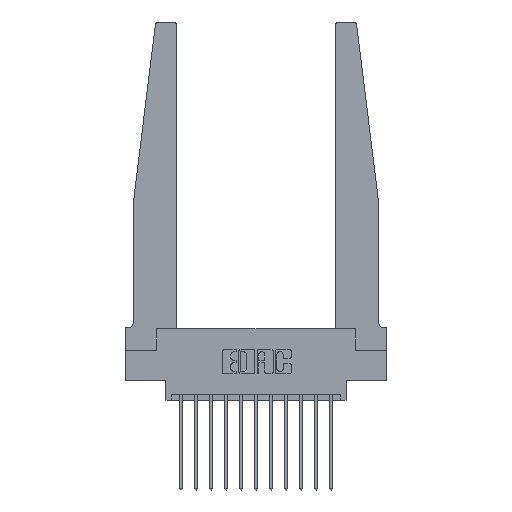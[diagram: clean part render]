
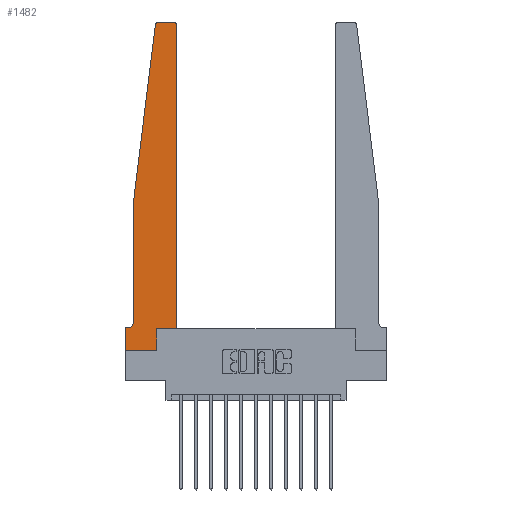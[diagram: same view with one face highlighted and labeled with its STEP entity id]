
A CAD part, top view. The second image highlights one B-rep face of the part: STEP entity #1482.
In plain terms, the highlighted planar face has unit normal (0, 0, 1).
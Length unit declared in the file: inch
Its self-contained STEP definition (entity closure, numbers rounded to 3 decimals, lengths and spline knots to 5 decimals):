
#38 = DIRECTION ( 'NONE',  ( 0., 0., 1. ) ) ;
#149 = ORIENTED_EDGE ( 'NONE', *, *, #4136, .T. ) ;
#203 = ORIENTED_EDGE ( 'NONE', *, *, #2887, .T. ) ;
#298 = ORIENTED_EDGE ( 'NONE', *, *, #16322, .T. ) ;
#369 = VECTOR ( 'NONE', #16697, 39.37008 ) ;
#582 = EDGE_CURVE ( 'NONE', #7267, #15739, #4285, .T. ) ;
#693 = EDGE_LOOP ( 'NONE', ( #4557, #298, #203, #1766, #14340, #6751, #10985, #16572, #149, #13660, #3062, #7093 ) ) ;
#736 = CIRCLE ( 'NONE', #2923, 0.05 ) ;
#879 = VERTEX_POINT ( 'NONE', #2829 ) ;
#1478 = CARTESIAN_POINT ( 'NONE',  ( 0.27653, 2.72, 0.37 ) ) ;
#1482 = ADVANCED_FACE ( 'NONE', ( #11853 ), #2599, .T. ) ;
#1578 = CARTESIAN_POINT ( 'NONE',  ( 0.24675, 2.72367, 0.37 ) ) ;
#1766 = ORIENTED_EDGE ( 'NONE', *, *, #582, .T. ) ;
#1962 = EDGE_CURVE ( 'NONE', #14315, #5229, #7698, .T. ) ;
#2391 = CARTESIAN_POINT ( 'NONE',  ( 0.015, 0.2375, 0.37 ) ) ;
#2501 = DIRECTION ( 'NONE',  ( 0., -1., 0. ) ) ;
#2599 = PLANE ( 'NONE',  #12465 ) ;
#2829 = CARTESIAN_POINT ( 'NONE',  ( 0.425, 0.18, 0.37 ) ) ;
#2849 = CARTESIAN_POINT ( 'NONE',  ( 0., 0.1875, 0.37 ) ) ;
#2887 = EDGE_CURVE ( 'NONE', #5390, #7267, #6261, .T. ) ;
#2923 = AXIS2_PLACEMENT_3D ( 'NONE', #2391, #7823, #10349 ) ;
#3027 = EDGE_CURVE ( 'NONE', #13052, #7630, #5092, .T. ) ;
#3062 = ORIENTED_EDGE ( 'NONE', *, *, #7537, .T. ) ;
#3632 = VERTEX_POINT ( 'NONE', #8326 ) ;
#3719 = LINE ( 'NONE', #8843, #8443 ) ;
#3731 = CARTESIAN_POINT ( 'NONE',  ( 0., 0., 0.37 ) ) ;
#4136 = EDGE_CURVE ( 'NONE', #5229, #7409, #14974, .T. ) ;
#4186 = DIRECTION ( 'NONE',  ( 0., 0., 1. ) ) ;
#4270 = CARTESIAN_POINT ( 'NONE',  ( 0.065, 0.1875, 0.37 ) ) ;
#4285 = LINE ( 'NONE', #14522, #10588 ) ;
#4311 = VECTOR ( 'NONE', #8189, 39.37008 ) ;
#4557 = ORIENTED_EDGE ( 'NONE', *, *, #11952, .T. ) ;
#4696 = CARTESIAN_POINT ( 'NONE',  ( 0.395, 2.75, 0.37 ) ) ;
#4885 = EDGE_CURVE ( 'NONE', #13196, #3632, #11730, .T. ) ;
#5019 = LINE ( 'NONE', #3731, #9753 ) ;
#5092 = CIRCLE ( 'NONE', #9356, 0.03 ) ;
#5199 = DIRECTION ( 'NONE',  ( 0., 0., 1. ) ) ;
#5229 = VERTEX_POINT ( 'NONE', #8824 ) ;
#5390 = VERTEX_POINT ( 'NONE', #1578 ) ;
#5505 = CARTESIAN_POINT ( 'NONE',  ( 0.425, 2.72, 0.37 ) ) ;
#6079 = CARTESIAN_POINT ( 'NONE',  ( 0., 0., 0.37 ) ) ;
#6261 = LINE ( 'NONE', #11383, #14456 ) ;
#6651 = DIRECTION ( 'NONE',  ( 0., 1., 0. ) ) ;
#6682 = DIRECTION ( 'NONE',  ( 1., 0., 0. ) ) ;
#6751 = ORIENTED_EDGE ( 'NONE', *, *, #4885, .T. ) ;
#6905 = CARTESIAN_POINT ( 'NONE',  ( 0.425, 0.18, 0.37 ) ) ;
#7093 = ORIENTED_EDGE ( 'NONE', *, *, #3027, .T. ) ;
#7267 = VERTEX_POINT ( 'NONE', #12842 ) ;
#7409 = VERTEX_POINT ( 'NONE', #8949 ) ;
#7537 = EDGE_CURVE ( 'NONE', #879, #13052, #15568, .T. ) ;
#7579 = CARTESIAN_POINT ( 'NONE',  ( 0.2605, 0.18, 0.37 ) ) ;
#7630 = VERTEX_POINT ( 'NONE', #4696 ) ;
#7698 = LINE ( 'NONE', #11559, #369 ) ;
#7778 = VECTOR ( 'NONE', #15057, 39.37008 ) ;
#7823 = DIRECTION ( 'NONE',  ( 0., 0., -1. ) ) ;
#8189 = DIRECTION ( 'NONE',  ( -1., 0., 0. ) ) ;
#8197 = VERTEX_POINT ( 'NONE', #10667 ) ;
#8326 = CARTESIAN_POINT ( 'NONE',  ( 0., 0.1875, 0.37 ) ) ;
#8443 = VECTOR ( 'NONE', #16583, 39.37008 ) ;
#8824 = CARTESIAN_POINT ( 'NONE',  ( 0.2605, 0., 0.37 ) ) ;
#8843 = CARTESIAN_POINT ( 'NONE',  ( 0.25, 2.75, 0.37 ) ) ;
#8949 = CARTESIAN_POINT ( 'NONE',  ( 0.2605, 0.18, 0.37 ) ) ;
#9166 = CARTESIAN_POINT ( 'NONE',  ( 0.425, 0.18, 0.37 ) ) ;
#9193 = CARTESIAN_POINT ( 'NONE',  ( 0.065, 0.2375, 0.37 ) ) ;
#9356 = AXIS2_PLACEMENT_3D ( 'NONE', #11712, #38, #6682 ) ;
#9753 = VECTOR ( 'NONE', #2501, 39.37008 ) ;
#10349 = DIRECTION ( 'NONE',  ( -1., 0., 0. ) ) ;
#10469 = CARTESIAN_POINT ( 'NONE',  ( 0.015, 0.1875, 0.37 ) ) ;
#10473 = EDGE_CURVE ( 'NONE', #7409, #879, #16117, .T. ) ;
#10588 = VECTOR ( 'NONE', #14607, 39.37008 ) ;
#10667 = CARTESIAN_POINT ( 'NONE',  ( 0.27653, 2.75, 0.37 ) ) ;
#10985 = ORIENTED_EDGE ( 'NONE', *, *, #14181, .T. ) ;
#11383 = CARTESIAN_POINT ( 'NONE',  ( 0.065, 1.25, 0.37 ) ) ;
#11405 = VECTOR ( 'NONE', #14790, 39.37008 ) ;
#11559 = CARTESIAN_POINT ( 'NONE',  ( 0., 0., 0.37 ) ) ;
#11643 = DIRECTION ( 'NONE',  ( 1., 0., 0. ) ) ;
#11712 = CARTESIAN_POINT ( 'NONE',  ( 0.395, 2.72, 0.37 ) ) ;
#11730 = LINE ( 'NONE', #4270, #4311 ) ;
#11853 = FACE_OUTER_BOUND ( 'NONE', #693, .T. ) ;
#11952 = EDGE_CURVE ( 'NONE', #7630, #8197, #3719, .T. ) ;
#12465 = AXIS2_PLACEMENT_3D ( 'NONE', #2849, #5199, #15439 ) ;
#12720 = CIRCLE ( 'NONE', #14865, 0.03 ) ;
#12842 = CARTESIAN_POINT ( 'NONE',  ( 0.065, 1.25, 0.37 ) ) ;
#12904 = EDGE_CURVE ( 'NONE', #15739, #13196, #736, .T. ) ;
#13052 = VERTEX_POINT ( 'NONE', #5505 ) ;
#13196 = VERTEX_POINT ( 'NONE', #10469 ) ;
#13660 = ORIENTED_EDGE ( 'NONE', *, *, #10473, .T. ) ;
#14181 = EDGE_CURVE ( 'NONE', #3632, #14315, #5019, .T. ) ;
#14315 = VERTEX_POINT ( 'NONE', #6079 ) ;
#14340 = ORIENTED_EDGE ( 'NONE', *, *, #12904, .T. ) ;
#14456 = VECTOR ( 'NONE', #16509, 39.37008 ) ;
#14522 = CARTESIAN_POINT ( 'NONE',  ( 0.065, 1.25, 0.37 ) ) ;
#14607 = DIRECTION ( 'NONE',  ( 0., -1., 0. ) ) ;
#14790 = DIRECTION ( 'NONE',  ( 1., 0., 0. ) ) ;
#14865 = AXIS2_PLACEMENT_3D ( 'NONE', #1478, #4186, #11643 ) ;
#14974 = LINE ( 'NONE', #7579, #7778 ) ;
#15057 = DIRECTION ( 'NONE',  ( 0., 1., 0. ) ) ;
#15439 = DIRECTION ( 'NONE',  ( 1., 0., 0. ) ) ;
#15568 = LINE ( 'NONE', #9166, #16387 ) ;
#15739 = VERTEX_POINT ( 'NONE', #9193 ) ;
#16117 = LINE ( 'NONE', #6905, #11405 ) ;
#16322 = EDGE_CURVE ( 'NONE', #8197, #5390, #12720, .T. ) ;
#16387 = VECTOR ( 'NONE', #6651, 39.37008 ) ;
#16509 = DIRECTION ( 'NONE',  ( -0.122, -0.992, 0. ) ) ;
#16572 = ORIENTED_EDGE ( 'NONE', *, *, #1962, .T. ) ;
#16583 = DIRECTION ( 'NONE',  ( -1., 0., 0. ) ) ;
#16697 = DIRECTION ( 'NONE',  ( 1., 0., 0. ) ) ;
